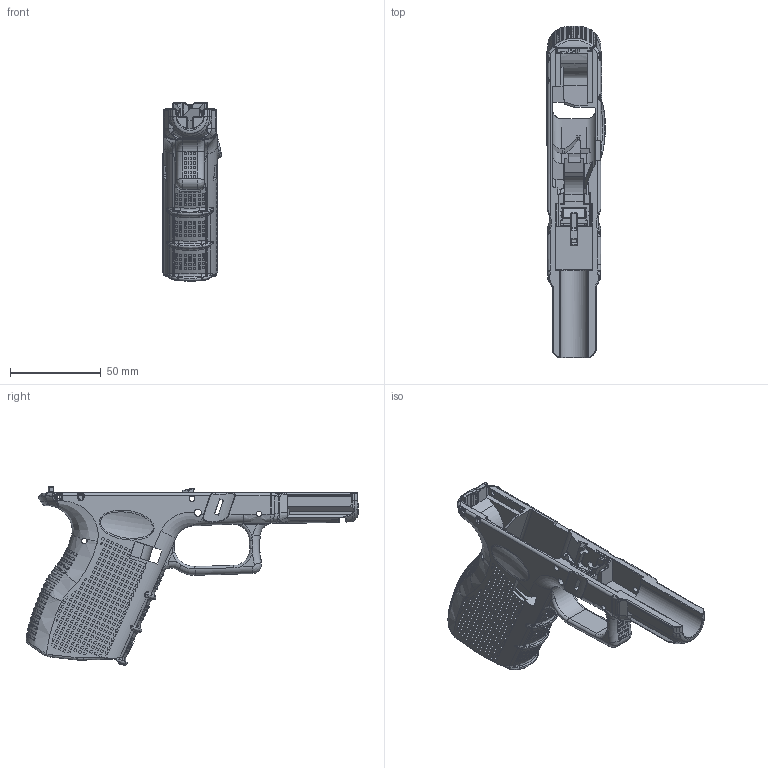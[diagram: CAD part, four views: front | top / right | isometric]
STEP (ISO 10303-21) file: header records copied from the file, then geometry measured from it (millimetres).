
FILE_DESCRIPTION(/* description */ (''),/* implementation_level */ '2;1');
FILE_NAME(/* name */ 'G19 oem grip.step',/* time_stamp */ '2019-08-09T20:34:11-07:00',/* author */ (''),/* organization */ (''),/* preprocessor_version */ 'ST-DEVELOPER v18',/* originating_system */ 'Autodesk Translation Framework v8.2.0.1029',/* authorisation */ '');
FILE_SCHEMA (('AUTOMOTIVE_DESIGN { 1 0 10303 214 3 1 1 }'));
Length unit declared in the file: millimetre
Products named in the file (1): G19 oem grip
Bounding box: 32.28 x 182.46 x 97.96 mm (x, y, z)
Volume: 83609.2 mm3; surface area: 48498.2 mm2
Topology: 1 solids, 2 shells, 5373 faces, 13364 edges, 8697 vertices
Faces by surface type: plane 4132, bspline 700, cylinder 411, torus 80, sphere 30, cone 20
Full cylindrical faces by diameter (mm): 2.4 x4, 2.997 x2, 3 x2, 3.175 x2, 3.962 x2
Entity records: 205711 total; most frequent: CARTESIAN_POINT 80485, ORIENTED_EDGE 26636, DIRECTION 23823, EDGE_CURVE 13318, LINE 9297, VECTOR 9297, VERTEX_POINT 8697, AXIS2_PLACEMENT_3D 7263
